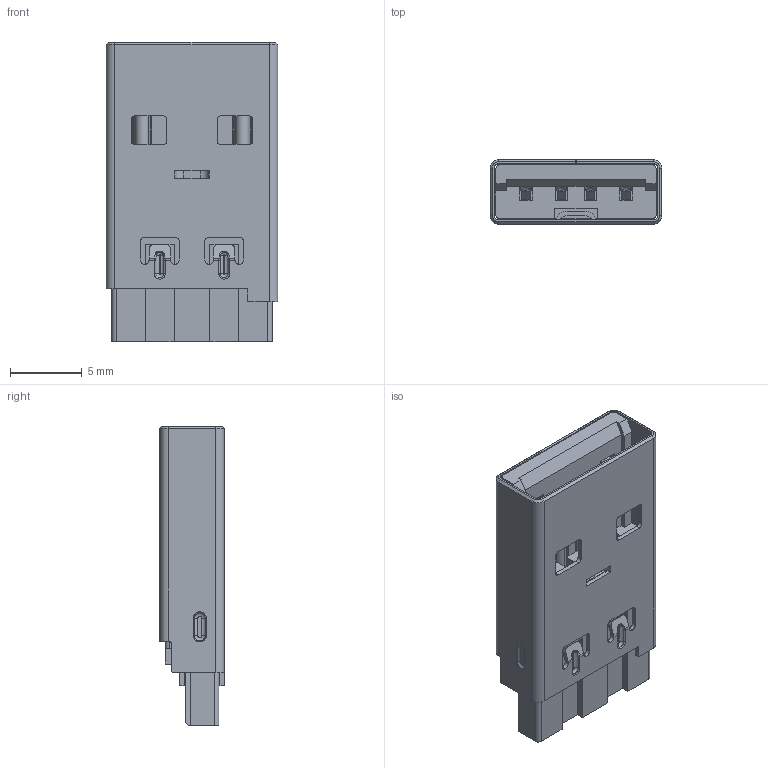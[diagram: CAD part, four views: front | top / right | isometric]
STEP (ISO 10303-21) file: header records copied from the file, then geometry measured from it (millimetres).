
FILE_DESCRIPTION (( 'STEP AP214' ), '1' );
FILE_NAME ('691C104-190-121.STEP', '2021-01-19T14:43:59', ( '' ), ( '' ), 'SwSTEP 2.0', 'SolidWorks 2020', '' );
FILE_SCHEMA (( 'AUTOMOTIVE_DESIGN' ));
Length unit declared in the file: millimetre
Products named in the file (5): Insulator 691C104-X90-12X_Black; Contact 2 691C104-X90-12X; Shell 691C104-X90-12X; 691C104-190-121; Contact 1 691C104-X90-12X
Assembly tree (6 placements, depth 2):
  691C104-190-121
    Shell 691C104-X90-12X
    Contact 2 691C104-X90-12X  x2
    Insulator 691C104-X90-12X_Black
    Contact 1 691C104-X90-12X  x2
Bounding box: 12 x 4.5 x 20.9 mm (x, y, z)
Volume: 630.1 mm3; surface area: 2246.7 mm2
Topology: 6 solids, 6 shells, 999 faces, 2525 edges, 1492 vertices
Faces by surface type: plane 476, bspline 317, cylinder 202, cone 4
Entity records: 28129 total; most frequent: CARTESIAN_POINT 12925, ORIENTED_EDGE 3522, DIRECTION 2520, EDGE_CURVE 1761, VERTEX_POINT 1072, VECTOR 1018, LINE 1018, AXIS2_PLACEMENT_3D 751
